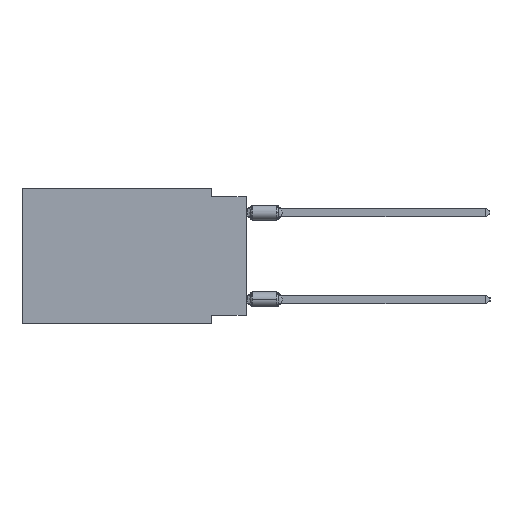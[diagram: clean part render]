
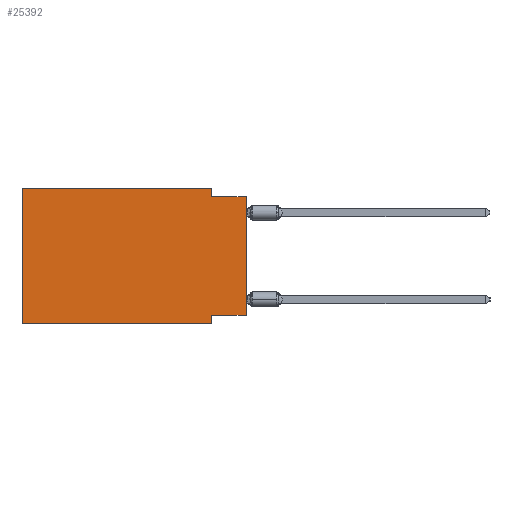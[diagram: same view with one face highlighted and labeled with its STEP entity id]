
A CAD part, left-side view. The second image highlights one B-rep face of the part: STEP entity #25392.
In plain terms, the highlighted planar face has unit normal (-1, 0, 0).
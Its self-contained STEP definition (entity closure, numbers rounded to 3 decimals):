
#937 = LINE ( 'NONE', #32905, #16875 ) ;
#955 = DIRECTION ( 'NONE',  ( 0., 0., -1. ) ) ;
#1098 = DIRECTION ( 'NONE',  ( 0., 0., -1. ) ) ;
#1640 = ORIENTED_EDGE ( 'NONE', *, *, #27439, .T. ) ;
#1903 = CARTESIAN_POINT ( 'NONE',  ( 0., 2.54, -0.635 ) ) ;
#2287 = ORIENTED_EDGE ( 'NONE', *, *, #10696, .F. ) ;
#2519 = EDGE_CURVE ( 'NONE', #4682, #33211, #9210, .T. ) ;
#2827 = CARTESIAN_POINT ( 'NONE',  ( 0., 0., -0.635 ) ) ;
#4682 = VERTEX_POINT ( 'NONE', #26355 ) ;
#6095 = PLANE ( 'NONE',  #7160 ) ;
#6098 = ORIENTED_EDGE ( 'NONE', *, *, #29391, .F. ) ;
#6572 = CARTESIAN_POINT ( 'NONE',  ( 0., 2.54, 0. ) ) ;
#7025 = LINE ( 'NONE', #25571, #19318 ) ;
#7160 = AXIS2_PLACEMENT_3D ( 'NONE', #19478, #32205, #1098 ) ;
#7248 = CARTESIAN_POINT ( 'NONE',  ( 0., 0., -0.635 ) ) ;
#8222 = VECTOR ( 'NONE', #22512, 1000. ) ;
#9210 = LINE ( 'NONE', #33093, #11259 ) ;
#10098 = DIRECTION ( 'NONE',  ( 0., 1., 0. ) ) ;
#10696 = EDGE_CURVE ( 'NONE', #29964, #21267, #31555, .T. ) ;
#11259 = VECTOR ( 'NONE', #955, 1000. ) ;
#11864 = ORIENTED_EDGE ( 'NONE', *, *, #26449, .F. ) ;
#12673 = CARTESIAN_POINT ( 'NONE',  ( 0., 0., -9.271 ) ) ;
#13311 = ORIENTED_EDGE ( 'NONE', *, *, #18836, .F. ) ;
#13416 = VERTEX_POINT ( 'NONE', #6572 ) ;
#14766 = VERTEX_POINT ( 'NONE', #1903 ) ;
#16509 = VECTOR ( 'NONE', #10098, 1000. ) ;
#16875 = VECTOR ( 'NONE', #27236, 1000. ) ;
#16956 = EDGE_LOOP ( 'NONE', ( #18652, #13311, #30497, #6098, #2287, #1640, #21904, #11864 ) ) ;
#17166 = VECTOR ( 'NONE', #33799, 1000. ) ;
#18403 = VERTEX_POINT ( 'NONE', #24908 ) ;
#18451 = CARTESIAN_POINT ( 'NONE',  ( 0., 16.383, -9.906 ) ) ;
#18652 = ORIENTED_EDGE ( 'NONE', *, *, #20285, .T. ) ;
#18836 = EDGE_CURVE ( 'NONE', #14766, #31083, #22873, .T. ) ;
#19146 = CARTESIAN_POINT ( 'NONE',  ( 0., 16.383, 0. ) ) ;
#19318 = VECTOR ( 'NONE', #19919, 1000. ) ;
#19478 = CARTESIAN_POINT ( 'NONE',  ( 0., 16.383, 0. ) ) ;
#19919 = DIRECTION ( 'NONE',  ( 0., -1., 0. ) ) ;
#20199 = CARTESIAN_POINT ( 'NONE',  ( 0., 2.54, -9.906 ) ) ;
#20234 = LINE ( 'NONE', #30712, #20565 ) ;
#20285 = EDGE_CURVE ( 'NONE', #18403, #31083, #937, .T. ) ;
#20565 = VECTOR ( 'NONE', #25547, 1000. ) ;
#20752 = LINE ( 'NONE', #12673, #16509 ) ;
#21267 = VERTEX_POINT ( 'NONE', #19146 ) ;
#21904 = ORIENTED_EDGE ( 'NONE', *, *, #2519, .F. ) ;
#22181 = LINE ( 'NONE', #22844, #8222 ) ;
#22512 = DIRECTION ( 'NONE',  ( 0., 0., -1. ) ) ;
#22844 = CARTESIAN_POINT ( 'NONE',  ( 0., 2.54, 0. ) ) ;
#22873 = LINE ( 'NONE', #7248, #23388 ) ;
#23388 = VECTOR ( 'NONE', #25446, 1000. ) ;
#24702 = EDGE_CURVE ( 'NONE', #13416, #14766, #22181, .T. ) ;
#24806 = FACE_OUTER_BOUND ( 'NONE', #16956, .T. ) ;
#24908 = CARTESIAN_POINT ( 'NONE',  ( 0., 0., -9.271 ) ) ;
#25392 = ADVANCED_FACE ( 'NONE', ( #24806 ), #6095, .F. ) ;
#25446 = DIRECTION ( 'NONE',  ( 0., -1., 0. ) ) ;
#25547 = DIRECTION ( 'NONE',  ( 0., -1., 0. ) ) ;
#25571 = CARTESIAN_POINT ( 'NONE',  ( 0., 16.383, -9.906 ) ) ;
#26355 = CARTESIAN_POINT ( 'NONE',  ( 0., 2.54, -9.271 ) ) ;
#26449 = EDGE_CURVE ( 'NONE', #18403, #4682, #20752, .T. ) ;
#27236 = DIRECTION ( 'NONE',  ( 0., 0., 1. ) ) ;
#27439 = EDGE_CURVE ( 'NONE', #29964, #33211, #7025, .T. ) ;
#28482 = CARTESIAN_POINT ( 'NONE',  ( 0., 16.383, 0. ) ) ;
#29391 = EDGE_CURVE ( 'NONE', #21267, #13416, #20234, .T. ) ;
#29964 = VERTEX_POINT ( 'NONE', #18451 ) ;
#30497 = ORIENTED_EDGE ( 'NONE', *, *, #24702, .F. ) ;
#30712 = CARTESIAN_POINT ( 'NONE',  ( 0., 16.383, 0. ) ) ;
#31083 = VERTEX_POINT ( 'NONE', #2827 ) ;
#31555 = LINE ( 'NONE', #28482, #17166 ) ;
#32205 = DIRECTION ( 'NONE',  ( 1., 0., 0. ) ) ;
#32905 = CARTESIAN_POINT ( 'NONE',  ( 0., 0., 0. ) ) ;
#33093 = CARTESIAN_POINT ( 'NONE',  ( 0., 2.54, -9.906 ) ) ;
#33211 = VERTEX_POINT ( 'NONE', #20199 ) ;
#33799 = DIRECTION ( 'NONE',  ( 0., 0., 1. ) ) ;
